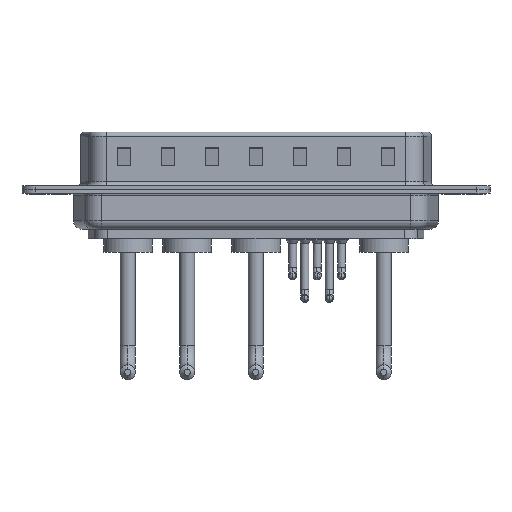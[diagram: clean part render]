
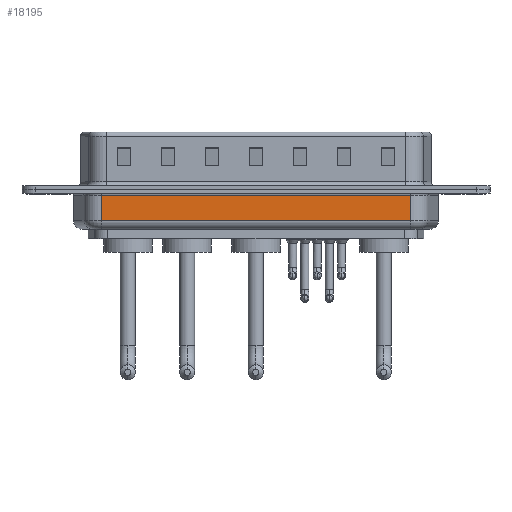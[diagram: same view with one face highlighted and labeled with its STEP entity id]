
A CAD part, front view. The second image highlights one B-rep face of the part: STEP entity #18195.
In plain terms, the highlighted planar face has unit normal (0, -1, 0).
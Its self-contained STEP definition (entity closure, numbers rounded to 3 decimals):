
#480 = EDGE_CURVE ( 'NONE', #9987, #1686, #9614, .T. ) ;
#559 = DIRECTION ( 'NONE',  ( 1., 0., 0. ) ) ;
#1686 = VERTEX_POINT ( 'NONE', #17244 ) ;
#2119 = VECTOR ( 'NONE', #18622, 1000. ) ;
#2479 = FACE_OUTER_BOUND ( 'NONE', #3965, .T. ) ;
#2602 = EDGE_CURVE ( 'NONE', #2761, #19993, #3509, .T. ) ;
#2761 = VERTEX_POINT ( 'NONE', #3928 ) ;
#2951 = CARTESIAN_POINT ( 'NONE',  ( 6.006, -5.35, -0.65 ) ) ;
#3509 = LINE ( 'NONE', #12988, #7260 ) ;
#3928 = CARTESIAN_POINT ( 'NONE',  ( 6.006, -5.35, -3.5 ) ) ;
#3965 = EDGE_LOOP ( 'NONE', ( #11839, #15057, #19870, #19806 ) ) ;
#5162 = LINE ( 'NONE', #11413, #7195 ) ;
#6282 = CARTESIAN_POINT ( 'NONE',  ( 6.006, -5.35, -0.65 ) ) ;
#7195 = VECTOR ( 'NONE', #559, 1000. ) ;
#7260 = VECTOR ( 'NONE', #14871, 1000. ) ;
#7665 = DIRECTION ( 'NONE',  ( -1., 0., 0. ) ) ;
#9237 = EDGE_CURVE ( 'NONE', #1686, #19993, #9241, .T. ) ;
#9241 = LINE ( 'NONE', #6282, #10356 ) ;
#9614 = LINE ( 'NONE', #20199, #2119 ) ;
#9987 = VERTEX_POINT ( 'NONE', #18470 ) ;
#10356 = VECTOR ( 'NONE', #7665, 1000. ) ;
#10411 = DIRECTION ( 'NONE',  ( 0., 0., 1. ) ) ;
#10889 = AXIS2_PLACEMENT_3D ( 'NONE', #11856, #15390, #10411 ) ;
#11413 = CARTESIAN_POINT ( 'NONE',  ( 6.006, -5.35, -3.5 ) ) ;
#11839 = ORIENTED_EDGE ( 'NONE', *, *, #2602, .F. ) ;
#11856 = CARTESIAN_POINT ( 'NONE',  ( 6.006, -5.35, -4.5 ) ) ;
#12274 = PLANE ( 'NONE',  #10889 ) ;
#12988 = CARTESIAN_POINT ( 'NONE',  ( 6.006, -5.35, -4.5 ) ) ;
#14871 = DIRECTION ( 'NONE',  ( 0., 0., 1. ) ) ;
#15057 = ORIENTED_EDGE ( 'NONE', *, *, #15601, .T. ) ;
#15390 = DIRECTION ( 'NONE',  ( 0., 1., 0. ) ) ;
#15601 = EDGE_CURVE ( 'NONE', #2761, #9987, #5162, .T. ) ;
#17244 = CARTESIAN_POINT ( 'NONE',  ( 41.044, -5.35, -0.65 ) ) ;
#18195 = ADVANCED_FACE ( 'NONE', ( #2479 ), #12274, .F. ) ;
#18470 = CARTESIAN_POINT ( 'NONE',  ( 41.044, -5.35, -3.5 ) ) ;
#18622 = DIRECTION ( 'NONE',  ( 0., 0., 1. ) ) ;
#19806 = ORIENTED_EDGE ( 'NONE', *, *, #9237, .T. ) ;
#19870 = ORIENTED_EDGE ( 'NONE', *, *, #480, .T. ) ;
#19993 = VERTEX_POINT ( 'NONE', #2951 ) ;
#20199 = CARTESIAN_POINT ( 'NONE',  ( 41.044, -5.35, -4.5 ) ) ;
